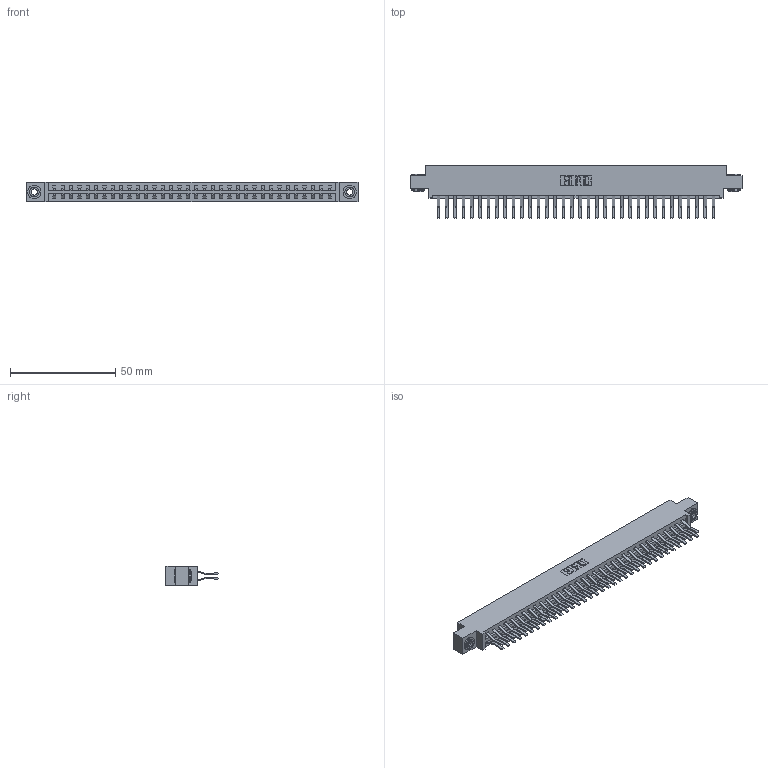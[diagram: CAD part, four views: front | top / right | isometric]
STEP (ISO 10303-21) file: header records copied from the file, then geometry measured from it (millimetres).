
FILE_DESCRIPTION (( 'STEP AP203' ), '1' );
FILE_NAME ('337-068-560-803.STEP', '2018-08-11T11:12:54', ( '' ), ( '' ), 'SwSTEP 2.0', 'SolidWorks 2016', '' );
FILE_SCHEMA (( 'CONFIG_CONTROL_DESIGN' ));
Length unit declared in the file: inch
Products named in the file (4): 337 Part_0.170 Offset - 0.156 Dia-TH; 345-292-001_560 Tail; 345-250-002_345-250-002-102; 337-068-560-803
Assembly tree (71 placements, depth 2):
  337-068-560-803
    337 Part_0.170 Offset - 0.156 Dia-TH
    345-292-001_560 Tail  x68
    345-250-002_345-250-002-102  x2
Bounding box: 157.73 x 24.78 x 9.4 mm (x, y, z)
Volume: 16864.4 mm3; surface area: 20609.7 mm2
Topology: 71 solids, 71 shells, 3964 faces, 11755 edges, 7742 vertices
Faces by surface type: plane 2668, cylinder 1288, cone 8
Entity records: 28266 total; most frequent: CARTESIAN_POINT 4745, ORIENTED_EDGE 4674, DIRECTION 4087, EDGE_CURVE 2337, LINE 2181, VECTOR 2181, VERTEX_POINT 1554, AXIS2_PLACEMENT_3D 953
